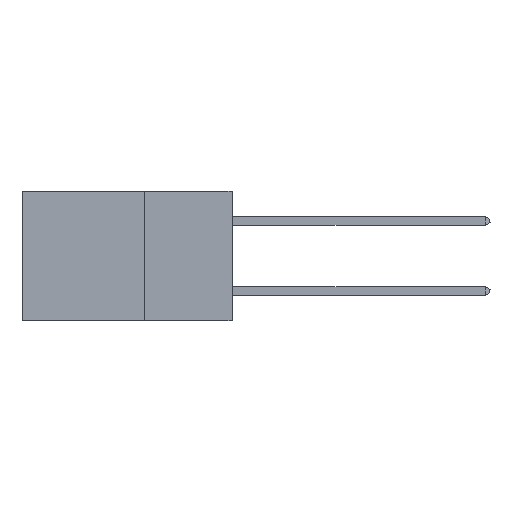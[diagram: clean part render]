
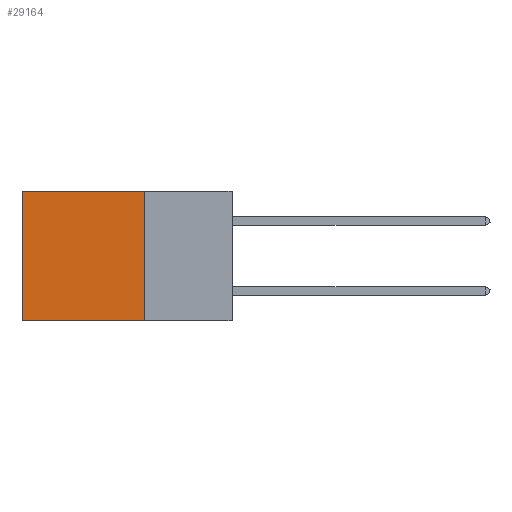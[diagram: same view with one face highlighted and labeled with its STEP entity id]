
A CAD part, left-side view. The second image highlights one B-rep face of the part: STEP entity #29164.
In plain terms, the highlighted planar face has unit normal (-1, 0, 0).
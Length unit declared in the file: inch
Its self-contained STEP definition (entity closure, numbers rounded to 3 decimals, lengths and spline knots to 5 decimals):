
#307 = VERTEX_POINT ( 'NONE', #36272 ) ;
#571 = ORIENTED_EDGE ( 'NONE', *, *, #33680, .F. ) ;
#1177 = VECTOR ( 'NONE', #11738, 39.37008 ) ;
#3963 = LINE ( 'NONE', #30153, #10745 ) ;
#5431 = VECTOR ( 'NONE', #20714, 39.37008 ) ;
#6329 = CARTESIAN_POINT ( 'NONE',  ( 0.2875, 0.25, 0. ) ) ;
#7020 = DIRECTION ( 'NONE',  ( 0., 0., -1. ) ) ;
#7829 = DIRECTION ( 'NONE',  ( 0., 0., -1. ) ) ;
#9968 = DIRECTION ( 'NONE',  ( 0., 1., 0. ) ) ;
#10454 = AXIS2_PLACEMENT_3D ( 'NONE', #12691, #24299, #7020 ) ;
#10724 = VERTEX_POINT ( 'NONE', #22044 ) ;
#10745 = VECTOR ( 'NONE', #9968, 39.37008 ) ;
#11738 = DIRECTION ( 'NONE',  ( 0., 1., 0. ) ) ;
#12691 = CARTESIAN_POINT ( 'NONE',  ( 0.2875, 0.25, 0. ) ) ;
#13018 = VECTOR ( 'NONE', #7829, 39.37008 ) ;
#13068 = LINE ( 'NONE', #6329, #5431 ) ;
#15154 = EDGE_CURVE ( 'NONE', #10724, #15426, #3963, .T. ) ;
#15426 = VERTEX_POINT ( 'NONE', #16949 ) ;
#15747 = LINE ( 'NONE', #30896, #13018 ) ;
#16949 = CARTESIAN_POINT ( 'NONE',  ( 0.2875, 0.6, -0.37 ) ) ;
#17485 = LINE ( 'NONE', #31926, #1177 ) ;
#18526 = PLANE ( 'NONE',  #10454 ) ;
#19558 = ORIENTED_EDGE ( 'NONE', *, *, #21076, .T. ) ;
#19722 = FACE_OUTER_BOUND ( 'NONE', #29013, .T. ) ;
#20686 = VERTEX_POINT ( 'NONE', #20720 ) ;
#20714 = DIRECTION ( 'NONE',  ( 0., 0., -1. ) ) ;
#20720 = CARTESIAN_POINT ( 'NONE',  ( 0.2875, 0.6, 0. ) ) ;
#21076 = EDGE_CURVE ( 'NONE', #20686, #15426, #15747, .T. ) ;
#22044 = CARTESIAN_POINT ( 'NONE',  ( 0.2875, 0.25, -0.37 ) ) ;
#22106 = ORIENTED_EDGE ( 'NONE', *, *, #15154, .F. ) ;
#24299 = DIRECTION ( 'NONE',  ( 1., 0., 0. ) ) ;
#25660 = EDGE_CURVE ( 'NONE', #307, #20686, #17485, .T. ) ;
#27261 = ORIENTED_EDGE ( 'NONE', *, *, #25660, .T. ) ;
#29013 = EDGE_LOOP ( 'NONE', ( #19558, #22106, #571, #27261 ) ) ;
#29164 = ADVANCED_FACE ( 'NONE', ( #19722 ), #18526, .F. ) ;
#30153 = CARTESIAN_POINT ( 'NONE',  ( 0.2875, 0.25, -0.37 ) ) ;
#30896 = CARTESIAN_POINT ( 'NONE',  ( 0.2875, 0.6, 0. ) ) ;
#31926 = CARTESIAN_POINT ( 'NONE',  ( 0.2875, 0.25, 0. ) ) ;
#33680 = EDGE_CURVE ( 'NONE', #307, #10724, #13068, .T. ) ;
#36272 = CARTESIAN_POINT ( 'NONE',  ( 0.2875, 0.25, 0. ) ) ;
